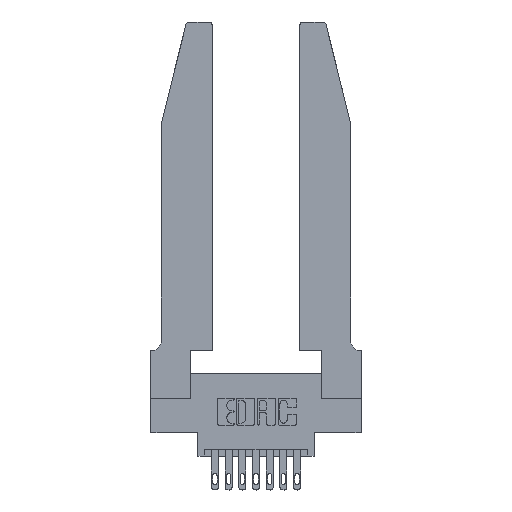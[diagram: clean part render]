
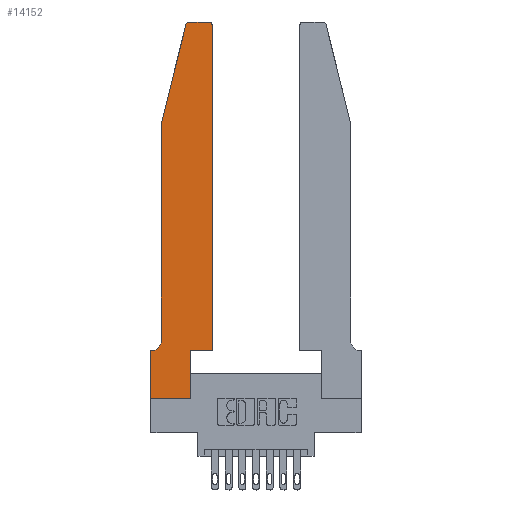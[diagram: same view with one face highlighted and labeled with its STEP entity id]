
A CAD part, top view. The second image highlights one B-rep face of the part: STEP entity #14152.
In plain terms, the highlighted planar face has unit normal (0, 0, 1).
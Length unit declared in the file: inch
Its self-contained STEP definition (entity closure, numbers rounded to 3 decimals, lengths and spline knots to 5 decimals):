
#92 = VERTEX_POINT ( 'NONE', #4015 ) ;
#216 = VERTEX_POINT ( 'NONE', #14841 ) ;
#389 = AXIS2_PLACEMENT_3D ( 'NONE', #4752, #12907, #5911 ) ;
#523 = CARTESIAN_POINT ( 'NONE',  ( 0.4505, 0.35, 0.37 ) ) ;
#532 = CARTESIAN_POINT ( 'NONE',  ( 0.4205, 2.72, 0.37 ) ) ;
#678 = CARTESIAN_POINT ( 'NONE',  ( 0.0755, 2., 0.37 ) ) ;
#712 = VERTEX_POINT ( 'NONE', #3701 ) ;
#892 = VERTEX_POINT ( 'NONE', #13613 ) ;
#905 = CARTESIAN_POINT ( 'NONE',  ( 0.4505, 0.35, 0.37 ) ) ;
#1206 = CARTESIAN_POINT ( 'NONE',  ( 0.4505, 0.35, 0.37 ) ) ;
#1516 = CARTESIAN_POINT ( 'NONE',  ( 0., 0., 0.37 ) ) ;
#1535 = CARTESIAN_POINT ( 'NONE',  ( 0.4205, 2.75, 0.37 ) ) ;
#1649 = EDGE_CURVE ( 'NONE', #10117, #14129, #10795, .T. ) ;
#1654 = LINE ( 'NONE', #14011, #10699 ) ;
#1729 = VECTOR ( 'NONE', #2616, 39.37008 ) ;
#1929 = FACE_OUTER_BOUND ( 'NONE', #13060, .T. ) ;
#1971 = DIRECTION ( 'NONE',  ( -1., 0., 0. ) ) ;
#1996 = EDGE_CURVE ( 'NONE', #14129, #92, #2259, .T. ) ;
#2051 = EDGE_CURVE ( 'NONE', #5078, #14901, #4906, .T. ) ;
#2187 = ORIENTED_EDGE ( 'NONE', *, *, #13357, .T. ) ;
#2259 = LINE ( 'NONE', #10664, #4412 ) ;
#2310 = EDGE_CURVE ( 'NONE', #5219, #712, #4743, .T. ) ;
#2616 = DIRECTION ( 'NONE',  ( 1., 0., 0. ) ) ;
#2853 = CARTESIAN_POINT ( 'NONE',  ( 0.2865, 0.35, 0.37 ) ) ;
#2954 = DIRECTION ( 'NONE',  ( 0., 0., 1. ) ) ;
#3267 = EDGE_CURVE ( 'NONE', #92, #892, #12786, .T. ) ;
#3314 = ORIENTED_EDGE ( 'NONE', *, *, #8245, .T. ) ;
#3510 = ORIENTED_EDGE ( 'NONE', *, *, #1649, .T. ) ;
#3701 = CARTESIAN_POINT ( 'NONE',  ( 0.2865, 0., 0.37 ) ) ;
#3750 = DIRECTION ( 'NONE',  ( -1., 0., 0. ) ) ;
#3916 = VECTOR ( 'NONE', #7862, 39.37008 ) ;
#4015 = CARTESIAN_POINT ( 'NONE',  ( 0.284, 2.75, 0.37 ) ) ;
#4245 = CARTESIAN_POINT ( 'NONE',  ( 0., 0.35, 0.37 ) ) ;
#4273 = DIRECTION ( 'NONE',  ( 1., 0., 0. ) ) ;
#4310 = ORIENTED_EDGE ( 'NONE', *, *, #2310, .T. ) ;
#4412 = VECTOR ( 'NONE', #3750, 39.37008 ) ;
#4743 = LINE ( 'NONE', #6165, #1729 ) ;
#4752 = CARTESIAN_POINT ( 'NONE',  ( 0.284, 2.72, 0.37 ) ) ;
#4772 = AXIS2_PLACEMENT_3D ( 'NONE', #6629, #6516, #1971 ) ;
#4906 = LINE ( 'NONE', #905, #13859 ) ;
#5078 = VERTEX_POINT ( 'NONE', #2853 ) ;
#5219 = VERTEX_POINT ( 'NONE', #12697 ) ;
#5250 = CARTESIAN_POINT ( 'NONE',  ( 0.0055, 0.35, 0.37 ) ) ;
#5289 = VERTEX_POINT ( 'NONE', #4245 ) ;
#5375 = DIRECTION ( 'NONE',  ( 1., 0., 0. ) ) ;
#5523 = VECTOR ( 'NONE', #14112, 39.37008 ) ;
#5911 = DIRECTION ( 'NONE',  ( 1., 0., 0. ) ) ;
#6043 = ORIENTED_EDGE ( 'NONE', *, *, #12797, .T. ) ;
#6165 = CARTESIAN_POINT ( 'NONE',  ( 0., 0., 0.37 ) ) ;
#6172 = DIRECTION ( 'NONE',  ( 0., 0., 1. ) ) ;
#6516 = DIRECTION ( 'NONE',  ( 0., 0., -1. ) ) ;
#6552 = ORIENTED_EDGE ( 'NONE', *, *, #2051, .T. ) ;
#6629 = CARTESIAN_POINT ( 'NONE',  ( 0.0055, 0.42, 0.37 ) ) ;
#6654 = ORIENTED_EDGE ( 'NONE', *, *, #10095, .T. ) ;
#6738 = LINE ( 'NONE', #12640, #14949 ) ;
#6761 = ORIENTED_EDGE ( 'NONE', *, *, #14712, .T. ) ;
#6984 = LINE ( 'NONE', #523, #5523 ) ;
#7327 = ORIENTED_EDGE ( 'NONE', *, *, #1996, .T. ) ;
#7398 = CARTESIAN_POINT ( 'NONE',  ( 0.0755, 2., 0.37 ) ) ;
#7862 = DIRECTION ( 'NONE',  ( 0., 1., 0. ) ) ;
#8245 = EDGE_CURVE ( 'NONE', #9259, #5289, #1654, .T. ) ;
#8471 = CIRCLE ( 'NONE', #4772, 0.07 ) ;
#8586 = ORIENTED_EDGE ( 'NONE', *, *, #9588, .T. ) ;
#8626 = LINE ( 'NONE', #1516, #14076 ) ;
#8737 = DIRECTION ( 'NONE',  ( 1., 0., 0. ) ) ;
#9259 = VERTEX_POINT ( 'NONE', #5250 ) ;
#9582 = VERTEX_POINT ( 'NONE', #678 ) ;
#9588 = EDGE_CURVE ( 'NONE', #216, #9259, #8471, .T. ) ;
#9600 = DIRECTION ( 'NONE',  ( 0., -1., 0. ) ) ;
#9630 = CARTESIAN_POINT ( 'NONE',  ( 0.2865, 0.35, 0.37 ) ) ;
#9955 = DIRECTION ( 'NONE',  ( 0., -1., 0. ) ) ;
#9973 = PLANE ( 'NONE',  #13140 ) ;
#10095 = EDGE_CURVE ( 'NONE', #14901, #10117, #6984, .T. ) ;
#10117 = VERTEX_POINT ( 'NONE', #10878 ) ;
#10477 = DIRECTION ( 'NONE',  ( -1., 0., 0. ) ) ;
#10664 = CARTESIAN_POINT ( 'NONE',  ( 0.2605, 2.75, 0.37 ) ) ;
#10667 = VECTOR ( 'NONE', #9955, 39.37008 ) ;
#10699 = VECTOR ( 'NONE', #10477, 39.37008 ) ;
#10795 = CIRCLE ( 'NONE', #11206, 0.03 ) ;
#10878 = CARTESIAN_POINT ( 'NONE',  ( 0.4505, 2.72, 0.37 ) ) ;
#11046 = LINE ( 'NONE', #7398, #10667 ) ;
#11091 = EDGE_CURVE ( 'NONE', #5289, #5219, #8626, .T. ) ;
#11206 = AXIS2_PLACEMENT_3D ( 'NONE', #532, #2954, #8737 ) ;
#11983 = ORIENTED_EDGE ( 'NONE', *, *, #3267, .T. ) ;
#12376 = ORIENTED_EDGE ( 'NONE', *, *, #11091, .T. ) ;
#12540 = DIRECTION ( 'NONE',  ( -0.239, -0.971, 0. ) ) ;
#12640 = CARTESIAN_POINT ( 'NONE',  ( 0.0755, 2., 0.37 ) ) ;
#12697 = CARTESIAN_POINT ( 'NONE',  ( 0., 0., 0.37 ) ) ;
#12786 = CIRCLE ( 'NONE', #389, 0.03 ) ;
#12797 = EDGE_CURVE ( 'NONE', #9582, #216, #11046, .T. ) ;
#12828 = LINE ( 'NONE', #9630, #3916 ) ;
#12907 = DIRECTION ( 'NONE',  ( 0., 0., 1. ) ) ;
#13060 = EDGE_LOOP ( 'NONE', ( #7327, #11983, #6761, #6043, #8586, #3314, #12376, #4310, #2187, #6552, #6654, #3510 ) ) ;
#13140 = AXIS2_PLACEMENT_3D ( 'NONE', #13192, #6172, #5375 ) ;
#13192 = CARTESIAN_POINT ( 'NONE',  ( 0., 0.35, 0.37 ) ) ;
#13357 = EDGE_CURVE ( 'NONE', #712, #5078, #12828, .T. ) ;
#13613 = CARTESIAN_POINT ( 'NONE',  ( 0.25487, 2.72718, 0.37 ) ) ;
#13859 = VECTOR ( 'NONE', #4273, 39.37008 ) ;
#14011 = CARTESIAN_POINT ( 'NONE',  ( 0.0755, 0.35, 0.37 ) ) ;
#14076 = VECTOR ( 'NONE', #9600, 39.37008 ) ;
#14112 = DIRECTION ( 'NONE',  ( 0., 1., 0. ) ) ;
#14129 = VERTEX_POINT ( 'NONE', #1535 ) ;
#14152 = ADVANCED_FACE ( 'NONE', ( #1929 ), #9973, .T. ) ;
#14712 = EDGE_CURVE ( 'NONE', #892, #9582, #6738, .T. ) ;
#14841 = CARTESIAN_POINT ( 'NONE',  ( 0.0755, 0.42, 0.37 ) ) ;
#14901 = VERTEX_POINT ( 'NONE', #1206 ) ;
#14949 = VECTOR ( 'NONE', #12540, 39.37008 ) ;
